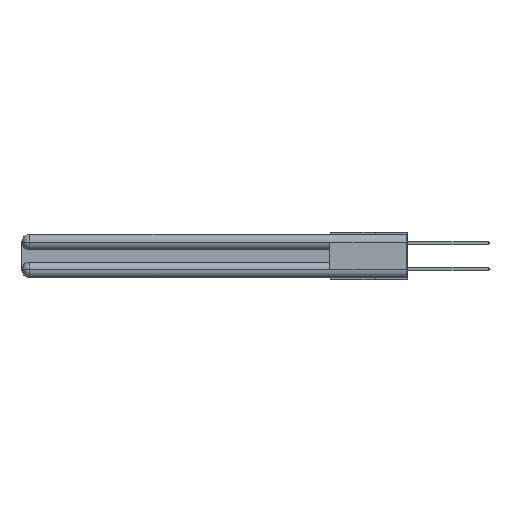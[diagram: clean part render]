
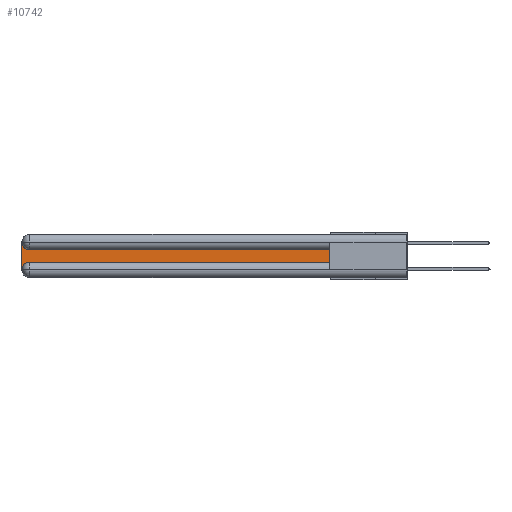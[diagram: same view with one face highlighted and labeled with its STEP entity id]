
A CAD part, left-side view. The second image highlights one B-rep face of the part: STEP entity #10742.
In plain terms, the highlighted planar face has unit normal (-1, 0, 0).
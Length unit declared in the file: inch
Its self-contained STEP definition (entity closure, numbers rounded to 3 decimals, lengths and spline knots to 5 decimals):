
#459 = VERTEX_POINT ( 'NONE', #32860 ) ;
#614 = VECTOR ( 'NONE', #19924, 39.37008 ) ;
#1734 = VERTEX_POINT ( 'NONE', #21130 ) ;
#2584 = CARTESIAN_POINT ( 'NONE',  ( 0.075, 0.6, -0.2175 ) ) ;
#3955 = DIRECTION ( 'NONE',  ( 0., 0., 1. ) ) ;
#3961 = DIRECTION ( 'NONE',  ( 0., -1., 0. ) ) ;
#4490 = ORIENTED_EDGE ( 'NONE', *, *, #27137, .T. ) ;
#4932 = DIRECTION ( 'NONE',  ( 0., 1., 0. ) ) ;
#5421 = FACE_OUTER_BOUND ( 'NONE', #26327, .T. ) ;
#6681 = AXIS2_PLACEMENT_3D ( 'NONE', #33772, #22843, #17608 ) ;
#6791 = EDGE_CURVE ( 'NONE', #24639, #459, #29925, .T. ) ;
#7358 = VERTEX_POINT ( 'NONE', #30451 ) ;
#8009 = ORIENTED_EDGE ( 'NONE', *, *, #29981, .T. ) ;
#9551 = EDGE_CURVE ( 'NONE', #7358, #24639, #26620, .T. ) ;
#9932 = CARTESIAN_POINT ( 'NONE',  ( 0.075, 2.94, -0.0625 ) ) ;
#10742 = ADVANCED_FACE ( 'NONE', ( #5421 ), #33761, .F. ) ;
#10953 = ORIENTED_EDGE ( 'NONE', *, *, #34996, .T. ) ;
#11813 = CIRCLE ( 'NONE', #6681, 0.06 ) ;
#11960 = VECTOR ( 'NONE', #3961, 39.37008 ) ;
#12229 = VECTOR ( 'NONE', #3955, 39.37008 ) ;
#12734 = DIRECTION ( 'NONE',  ( 1., 0., 0. ) ) ;
#12863 = DIRECTION ( 'NONE',  ( 0., 0., -1. ) ) ;
#13367 = ORIENTED_EDGE ( 'NONE', *, *, #9551, .T. ) ;
#13626 = VERTEX_POINT ( 'NONE', #29749 ) ;
#13981 = LINE ( 'NONE', #33664, #614 ) ;
#16783 = AXIS2_PLACEMENT_3D ( 'NONE', #9932, #12734, #12863 ) ;
#17236 = DIRECTION ( 'NONE',  ( 1., 0., 0. ) ) ;
#17608 = DIRECTION ( 'NONE',  ( 0., 0., -1. ) ) ;
#19665 = AXIS2_PLACEMENT_3D ( 'NONE', #33879, #17236, #30682 ) ;
#19924 = DIRECTION ( 'NONE',  ( 0., 0., -1. ) ) ;
#21130 = CARTESIAN_POINT ( 'NONE',  ( 0.075, 3., -0.2775 ) ) ;
#22843 = DIRECTION ( 'NONE',  ( 1., 0., 0. ) ) ;
#23888 = CARTESIAN_POINT ( 'NONE',  ( 0.075, 0.6, -0.2175 ) ) ;
#24179 = CIRCLE ( 'NONE', #16783, 0.06 ) ;
#24639 = VERTEX_POINT ( 'NONE', #2584 ) ;
#25140 = CARTESIAN_POINT ( 'NONE',  ( 0.075, 0.6, -0.2175 ) ) ;
#25169 = VERTEX_POINT ( 'NONE', #33887 ) ;
#25713 = VECTOR ( 'NONE', #4932, 39.37008 ) ;
#26327 = EDGE_LOOP ( 'NONE', ( #4490, #8009, #10953, #29582, #13367, #27671 ) ) ;
#26620 = LINE ( 'NONE', #25140, #11960 ) ;
#27137 = EDGE_CURVE ( 'NONE', #459, #25169, #33099, .T. ) ;
#27671 = ORIENTED_EDGE ( 'NONE', *, *, #6791, .T. ) ;
#27902 = EDGE_CURVE ( 'NONE', #1734, #7358, #11813, .T. ) ;
#29582 = ORIENTED_EDGE ( 'NONE', *, *, #27902, .T. ) ;
#29749 = CARTESIAN_POINT ( 'NONE',  ( 0.075, 3., -0.0625 ) ) ;
#29925 = LINE ( 'NONE', #23888, #12229 ) ;
#29981 = EDGE_CURVE ( 'NONE', #25169, #13626, #24179, .T. ) ;
#30451 = CARTESIAN_POINT ( 'NONE',  ( 0.075, 2.94, -0.2175 ) ) ;
#30682 = DIRECTION ( 'NONE',  ( 0., 0., -1. ) ) ;
#32860 = CARTESIAN_POINT ( 'NONE',  ( 0.075, 0.6, -0.1225 ) ) ;
#33099 = LINE ( 'NONE', #35598, #25713 ) ;
#33664 = CARTESIAN_POINT ( 'NONE',  ( 0.075, 3., -0.2175 ) ) ;
#33761 = PLANE ( 'NONE',  #19665 ) ;
#33772 = CARTESIAN_POINT ( 'NONE',  ( 0.075, 2.94, -0.2775 ) ) ;
#33879 = CARTESIAN_POINT ( 'NONE',  ( 0.075, 3., -0.1225 ) ) ;
#33887 = CARTESIAN_POINT ( 'NONE',  ( 0.075, 2.94, -0.1225 ) ) ;
#34996 = EDGE_CURVE ( 'NONE', #13626, #1734, #13981, .T. ) ;
#35598 = CARTESIAN_POINT ( 'NONE',  ( 0.075, 0.6, -0.1225 ) ) ;
